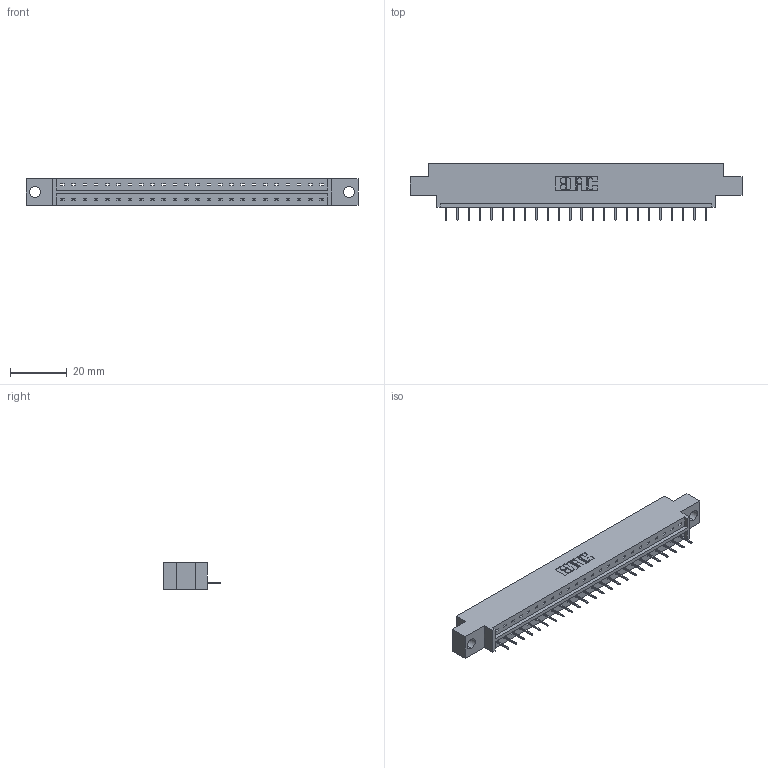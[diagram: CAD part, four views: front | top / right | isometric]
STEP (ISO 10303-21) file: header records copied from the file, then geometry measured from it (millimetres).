
FILE_DESCRIPTION (( 'STEP AP203' ), '1' );
FILE_NAME ('833-024-524-604.STEP', '2020-06-01T20:59:53', ( '' ), ( '' ), 'SwSTEP 2.0', 'SolidWorks 2020', '' );
FILE_SCHEMA (( 'CONFIG_CONTROL_DESIGN' ));
Length unit declared in the file: inch
Products named in the file (3): 833-024-524-604; 833 Part_Offset - .156 Dia - TH; 345-292-001_345-293-124
Assembly tree (25 placements, depth 2):
  833-024-524-604
    833 Part_Offset - .156 Dia - TH
    345-292-001_345-293-124  x24
Bounding box: 116.64 x 19.69 x 9.4 mm (x, y, z)
Volume: 11171.7 mm3; surface area: 11637.3 mm2
Topology: 25 solids, 25 shells, 1606 faces, 4643 edges, 2998 vertices
Faces by surface type: plane 1226, cylinder 380
Entity records: 17209 total; most frequent: CARTESIAN_POINT 2978, ORIENTED_EDGE 2938, DIRECTION 2549, EDGE_CURVE 1469, VECTOR 1345, LINE 1345, VERTEX_POINT 974, AXIS2_PLACEMENT_3D 602
